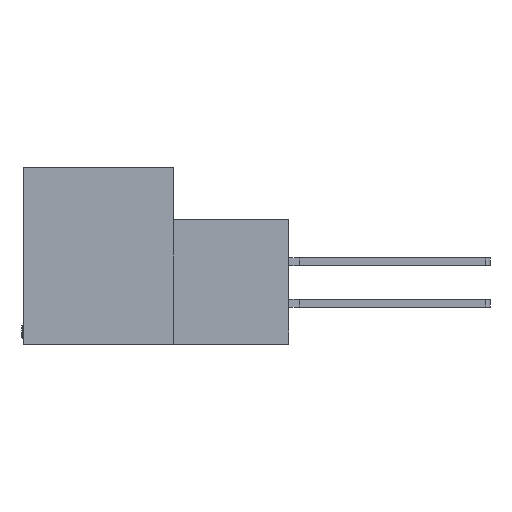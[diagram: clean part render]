
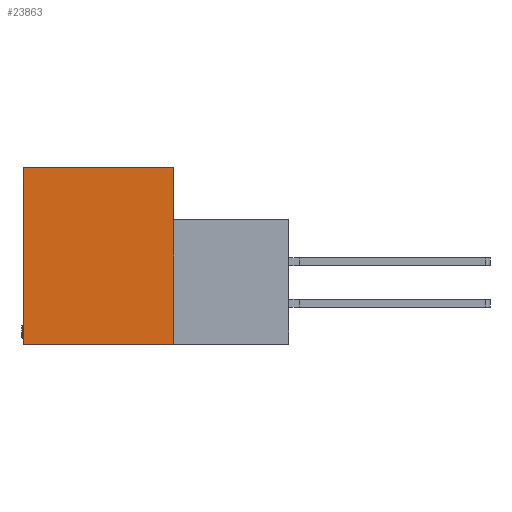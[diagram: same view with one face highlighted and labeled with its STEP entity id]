
A CAD part, left-side view. The second image highlights one B-rep face of the part: STEP entity #23863.
In plain terms, the highlighted planar face has unit normal (-1, 0, 0).
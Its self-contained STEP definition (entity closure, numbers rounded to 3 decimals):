
#66 = FACE_OUTER_BOUND ( 'NONE', #7842, .T. ) ;
#708 = CARTESIAN_POINT ( 'NONE',  ( 0., 0., 0. ) ) ;
#813 = CARTESIAN_POINT ( 'NONE',  ( 0., 0., 0. ) ) ;
#1391 = VECTOR ( 'NONE', #9362, 1000. ) ;
#2042 = ORIENTED_EDGE ( 'NONE', *, *, #17570, .F. ) ;
#2340 = DIRECTION ( 'NONE',  ( 0., 0., -1. ) ) ;
#2501 = ORIENTED_EDGE ( 'NONE', *, *, #7165, .F. ) ;
#4112 = CARTESIAN_POINT ( 'NONE',  ( 0., 11.506, 0. ) ) ;
#4599 = DIRECTION ( 'NONE',  ( 1., 0., 0. ) ) ;
#6662 = CARTESIAN_POINT ( 'NONE',  ( 0., -8.814, -13.487 ) ) ;
#7165 = EDGE_CURVE ( 'NONE', #8156, #19021, #16098, .T. ) ;
#7842 = EDGE_LOOP ( 'NONE', ( #2042, #21200, #2501, #13638 ) ) ;
#8156 = VERTEX_POINT ( 'NONE', #23221 ) ;
#9227 = AXIS2_PLACEMENT_3D ( 'NONE', #813, #4599, #12037 ) ;
#9362 = DIRECTION ( 'NONE',  ( 0., -1., 0. ) ) ;
#10201 = VECTOR ( 'NONE', #14137, 1000. ) ;
#10732 = VERTEX_POINT ( 'NONE', #20216 ) ;
#10740 = VECTOR ( 'NONE', #2340, 1000. ) ;
#11593 = DIRECTION ( 'NONE',  ( 0., 0., 1. ) ) ;
#11923 = EDGE_CURVE ( 'NONE', #18955, #8156, #20755, .T. ) ;
#12037 = DIRECTION ( 'NONE',  ( 0., 0., -1. ) ) ;
#13032 = CARTESIAN_POINT ( 'NONE',  ( 0., 0., 0. ) ) ;
#13354 = CARTESIAN_POINT ( 'NONE',  ( 0., 11.506, -13.487 ) ) ;
#13638 = ORIENTED_EDGE ( 'NONE', *, *, #11923, .F. ) ;
#14137 = DIRECTION ( 'NONE',  ( 0., 1., 0. ) ) ;
#15306 = VECTOR ( 'NONE', #11593, 1000. ) ;
#16098 = LINE ( 'NONE', #4112, #1391 ) ;
#16251 = LINE ( 'NONE', #6662, #10201 ) ;
#16772 = LINE ( 'NONE', #708, #10740 ) ;
#17570 = EDGE_CURVE ( 'NONE', #10732, #18955, #16251, .T. ) ;
#18669 = EDGE_CURVE ( 'NONE', #19021, #10732, #16772, .T. ) ;
#18955 = VERTEX_POINT ( 'NONE', #20071 ) ;
#19021 = VERTEX_POINT ( 'NONE', #13032 ) ;
#20071 = CARTESIAN_POINT ( 'NONE',  ( 0., 11.506, -13.487 ) ) ;
#20216 = CARTESIAN_POINT ( 'NONE',  ( 0., 0., -13.487 ) ) ;
#20755 = LINE ( 'NONE', #13354, #15306 ) ;
#21184 = PLANE ( 'NONE',  #9227 ) ;
#21200 = ORIENTED_EDGE ( 'NONE', *, *, #18669, .F. ) ;
#23221 = CARTESIAN_POINT ( 'NONE',  ( 0., 11.506, 0. ) ) ;
#23863 = ADVANCED_FACE ( 'NONE', ( #66 ), #21184, .F. ) ;
